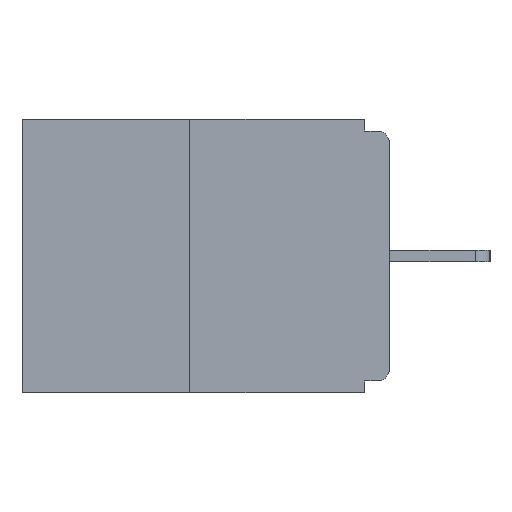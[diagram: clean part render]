
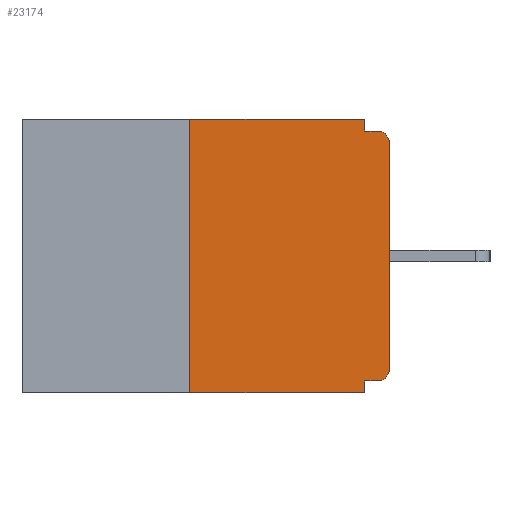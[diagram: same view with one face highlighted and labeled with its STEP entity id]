
A CAD part, left-side view. The second image highlights one B-rep face of the part: STEP entity #23174.
In plain terms, the highlighted planar face has unit normal (-1, 0, 0).
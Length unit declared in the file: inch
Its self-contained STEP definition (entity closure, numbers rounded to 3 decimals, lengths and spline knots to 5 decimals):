
#234 = DIRECTION ( 'NONE',  ( 0., -1., 0. ) ) ;
#444 = AXIS2_PLACEMENT_3D ( 'NONE', #17454, #19525, #15617 ) ;
#736 = DIRECTION ( 'NONE',  ( -1., 0., 0. ) ) ;
#747 = FACE_OUTER_BOUND ( 'NONE', #1350, .T. ) ;
#769 = EDGE_CURVE ( 'NONE', #12798, #9161, #9329, .T. ) ;
#1149 = DIRECTION ( 'NONE',  ( 0., 0., 1. ) ) ;
#1350 = EDGE_LOOP ( 'NONE', ( #21638, #8270, #2246, #2587, #6436, #21320, #18590, #11168, #11749, #1942 ) ) ;
#1402 = VERTEX_POINT ( 'NONE', #21898 ) ;
#1942 = ORIENTED_EDGE ( 'NONE', *, *, #5661, .F. ) ;
#2246 = ORIENTED_EDGE ( 'NONE', *, *, #769, .T. ) ;
#2587 = ORIENTED_EDGE ( 'NONE', *, *, #9658, .F. ) ;
#2822 = VECTOR ( 'NONE', #23956, 39.37008 ) ;
#2938 = EDGE_CURVE ( 'NONE', #12114, #16491, #15478, .T. ) ;
#4100 = VECTOR ( 'NONE', #23877, 39.37008 ) ;
#5085 = CARTESIAN_POINT ( 'NONE',  ( 0., 0., -0.015 ) ) ;
#5087 = DIRECTION ( 'NONE',  ( 0., 0., -1. ) ) ;
#5661 = EDGE_CURVE ( 'NONE', #16491, #20617, #18321, .T. ) ;
#5751 = DIRECTION ( 'NONE',  ( 0., -1., 0. ) ) ;
#6370 = CARTESIAN_POINT ( 'NONE',  ( 0., 0.015, -0.015 ) ) ;
#6436 = ORIENTED_EDGE ( 'NONE', *, *, #20476, .F. ) ;
#6927 = CARTESIAN_POINT ( 'NONE',  ( 0., 0.031, -0.343 ) ) ;
#7088 = EDGE_CURVE ( 'NONE', #12604, #14026, #17735, .T. ) ;
#8086 = CARTESIAN_POINT ( 'NONE',  ( 0., 0.015, -0.03 ) ) ;
#8270 = ORIENTED_EDGE ( 'NONE', *, *, #21670, .F. ) ;
#8602 = CARTESIAN_POINT ( 'NONE',  ( 0., 0.25, 0. ) ) ;
#9104 = LINE ( 'NONE', #16617, #9380 ) ;
#9161 = VERTEX_POINT ( 'NONE', #15957 ) ;
#9329 = LINE ( 'NONE', #20740, #10825 ) ;
#9380 = VECTOR ( 'NONE', #24089, 39.37008 ) ;
#9658 = EDGE_CURVE ( 'NONE', #14082, #9161, #14326, .T. ) ;
#9952 = PLANE ( 'NONE',  #444 ) ;
#10154 = VECTOR ( 'NONE', #21577, 39.37008 ) ;
#10501 = LINE ( 'NONE', #5085, #4100 ) ;
#10512 = CARTESIAN_POINT ( 'NONE',  ( 0., 0.25, -0.343 ) ) ;
#10825 = VECTOR ( 'NONE', #234, 39.37008 ) ;
#10962 = VECTOR ( 'NONE', #1149, 39.37008 ) ;
#11168 = ORIENTED_EDGE ( 'NONE', *, *, #20223, .T. ) ;
#11749 = ORIENTED_EDGE ( 'NONE', *, *, #17685, .F. ) ;
#11755 = CARTESIAN_POINT ( 'NONE',  ( 0., 0., -0.313 ) ) ;
#12114 = VERTEX_POINT ( 'NONE', #8602 ) ;
#12264 = VECTOR ( 'NONE', #5087, 39.37008 ) ;
#12601 = CARTESIAN_POINT ( 'NONE',  ( 0., 0.015, -0.313 ) ) ;
#12604 = VERTEX_POINT ( 'NONE', #11755 ) ;
#12798 = VERTEX_POINT ( 'NONE', #10512 ) ;
#13640 = VECTOR ( 'NONE', #5751, 39.37008 ) ;
#14026 = VERTEX_POINT ( 'NONE', #17522 ) ;
#14082 = VERTEX_POINT ( 'NONE', #18012 ) ;
#14308 = CARTESIAN_POINT ( 'NONE',  ( 0., 0., 0. ) ) ;
#14326 = LINE ( 'NONE', #6927, #12264 ) ;
#14442 = DIRECTION ( 'NONE',  ( 0., 0., -1. ) ) ;
#14518 = CARTESIAN_POINT ( 'NONE',  ( 0., 0.031, 0. ) ) ;
#14842 = CIRCLE ( 'NONE', #23472, 0.015 ) ;
#15106 = CARTESIAN_POINT ( 'NONE',  ( 0., 0.46, 0. ) ) ;
#15478 = LINE ( 'NONE', #15106, #13640 ) ;
#15617 = DIRECTION ( 'NONE',  ( 0., 0., -1. ) ) ;
#15957 = CARTESIAN_POINT ( 'NONE',  ( 0., 0.031, -0.343 ) ) ;
#16291 = DIRECTION ( 'NONE',  ( -1., 0., 0. ) ) ;
#16460 = AXIS2_PLACEMENT_3D ( 'NONE', #12601, #16291, #14442 ) ;
#16491 = VERTEX_POINT ( 'NONE', #22347 ) ;
#16549 = CARTESIAN_POINT ( 'NONE',  ( 0., 0.031, -0.015 ) ) ;
#16617 = CARTESIAN_POINT ( 'NONE',  ( 0., 0.25, 0. ) ) ;
#17454 = CARTESIAN_POINT ( 'NONE',  ( 0., 0.46, 0. ) ) ;
#17522 = CARTESIAN_POINT ( 'NONE',  ( 0., 0., -0.03 ) ) ;
#17618 = CIRCLE ( 'NONE', #16460, 0.015 ) ;
#17685 = EDGE_CURVE ( 'NONE', #20617, #20156, #10501, .T. ) ;
#17735 = LINE ( 'NONE', #14308, #10962 ) ;
#18012 = CARTESIAN_POINT ( 'NONE',  ( 0., 0.031, -0.328 ) ) ;
#18321 = LINE ( 'NONE', #14518, #2822 ) ;
#18590 = ORIENTED_EDGE ( 'NONE', *, *, #7088, .T. ) ;
#19525 = DIRECTION ( 'NONE',  ( 1., 0., 0. ) ) ;
#19617 = LINE ( 'NONE', #23432, #10154 ) ;
#20156 = VERTEX_POINT ( 'NONE', #6370 ) ;
#20223 = EDGE_CURVE ( 'NONE', #14026, #20156, #14842, .T. ) ;
#20476 = EDGE_CURVE ( 'NONE', #1402, #14082, #19617, .T. ) ;
#20617 = VERTEX_POINT ( 'NONE', #16549 ) ;
#20740 = CARTESIAN_POINT ( 'NONE',  ( 0., 0.46, -0.343 ) ) ;
#21089 = EDGE_CURVE ( 'NONE', #1402, #12604, #17618, .T. ) ;
#21320 = ORIENTED_EDGE ( 'NONE', *, *, #21089, .T. ) ;
#21577 = DIRECTION ( 'NONE',  ( 0., 1., 0. ) ) ;
#21638 = ORIENTED_EDGE ( 'NONE', *, *, #2938, .F. ) ;
#21670 = EDGE_CURVE ( 'NONE', #12798, #12114, #9104, .T. ) ;
#21898 = CARTESIAN_POINT ( 'NONE',  ( 0., 0.015, -0.328 ) ) ;
#22347 = CARTESIAN_POINT ( 'NONE',  ( 0., 0.031, 0. ) ) ;
#23174 = ADVANCED_FACE ( 'NONE', ( #747 ), #9952, .F. ) ;
#23328 = DIRECTION ( 'NONE',  ( 0., 0., -1. ) ) ;
#23432 = CARTESIAN_POINT ( 'NONE',  ( 0., 0., -0.328 ) ) ;
#23472 = AXIS2_PLACEMENT_3D ( 'NONE', #8086, #736, #23328 ) ;
#23877 = DIRECTION ( 'NONE',  ( 0., -1., 0. ) ) ;
#23956 = DIRECTION ( 'NONE',  ( 0., 0., -1. ) ) ;
#24089 = DIRECTION ( 'NONE',  ( 0., 0., 1. ) ) ;
